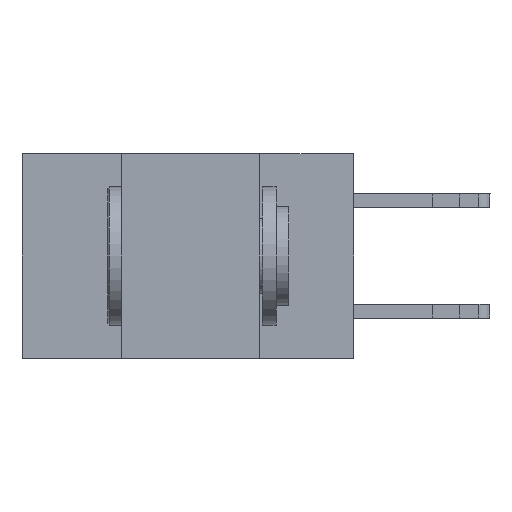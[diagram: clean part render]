
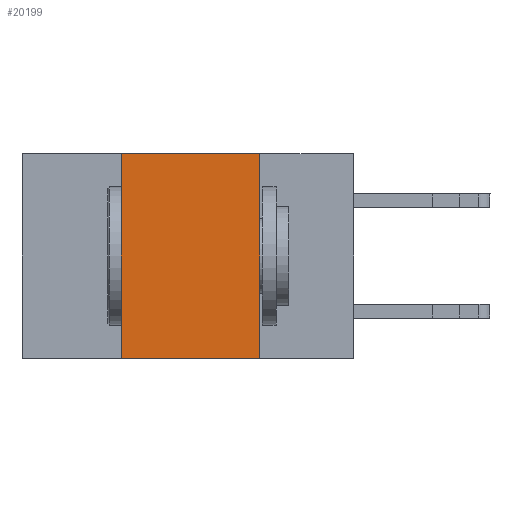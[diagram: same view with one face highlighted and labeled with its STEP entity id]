
A CAD part, left-side view. The second image highlights one B-rep face of the part: STEP entity #20199.
In plain terms, the highlighted planar face has unit normal (-1, 0, 0).
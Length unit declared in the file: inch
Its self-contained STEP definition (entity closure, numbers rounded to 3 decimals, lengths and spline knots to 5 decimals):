
#321 = PLANE ( 'NONE',  #13022 ) ;
#457 = CARTESIAN_POINT ( 'NONE',  ( 0., 0.17, -0.37 ) ) ;
#1459 = DIRECTION ( 'NONE',  ( 0., -1., 0. ) ) ;
#2272 = VERTEX_POINT ( 'NONE', #10767 ) ;
#2570 = DIRECTION ( 'NONE',  ( 1., 0., 0. ) ) ;
#2730 = CARTESIAN_POINT ( 'NONE',  ( 0., 0.17, 0. ) ) ;
#2956 = LINE ( 'NONE', #11340, #7273 ) ;
#3131 = LINE ( 'NONE', #12215, #18068 ) ;
#4416 = VECTOR ( 'NONE', #21089, 39.37008 ) ;
#4580 = EDGE_CURVE ( 'NONE', #12915, #20839, #3131, .T. ) ;
#4946 = CARTESIAN_POINT ( 'NONE',  ( 0., 0.42, 0. ) ) ;
#5567 = LINE ( 'NONE', #2730, #7060 ) ;
#6521 = CARTESIAN_POINT ( 'NONE',  ( 0., 0.6, 0. ) ) ;
#7060 = VECTOR ( 'NONE', #10227, 39.37008 ) ;
#7273 = VECTOR ( 'NONE', #1459, 39.37008 ) ;
#9674 = LINE ( 'NONE', #13425, #4416 ) ;
#9682 = CARTESIAN_POINT ( 'NONE',  ( 0., 0.42, -0.37 ) ) ;
#10227 = DIRECTION ( 'NONE',  ( 0., 0., -1. ) ) ;
#10244 = ORIENTED_EDGE ( 'NONE', *, *, #13950, .F. ) ;
#10767 = CARTESIAN_POINT ( 'NONE',  ( 0., 0.17, 0. ) ) ;
#11340 = CARTESIAN_POINT ( 'NONE',  ( 0., 0.6, 0. ) ) ;
#12215 = CARTESIAN_POINT ( 'NONE',  ( 0., 0.6, -0.37 ) ) ;
#12915 = VERTEX_POINT ( 'NONE', #9682 ) ;
#13022 = AXIS2_PLACEMENT_3D ( 'NONE', #6521, #2570, #19939 ) ;
#13425 = CARTESIAN_POINT ( 'NONE',  ( 0., 0.42, 0. ) ) ;
#13950 = EDGE_CURVE ( 'NONE', #19015, #2272, #2956, .T. ) ;
#14674 = EDGE_CURVE ( 'NONE', #12915, #19015, #9674, .T. ) ;
#14960 = ORIENTED_EDGE ( 'NONE', *, *, #18806, .F. ) ;
#18068 = VECTOR ( 'NONE', #21812, 39.37008 ) ;
#18806 = EDGE_CURVE ( 'NONE', #2272, #20839, #5567, .T. ) ;
#19015 = VERTEX_POINT ( 'NONE', #4946 ) ;
#19890 = EDGE_LOOP ( 'NONE', ( #14960, #10244, #24963, #21073 ) ) ;
#19939 = DIRECTION ( 'NONE',  ( 0., 0., -1. ) ) ;
#20199 = ADVANCED_FACE ( 'NONE', ( #21256 ), #321, .F. ) ;
#20839 = VERTEX_POINT ( 'NONE', #457 ) ;
#21073 = ORIENTED_EDGE ( 'NONE', *, *, #4580, .T. ) ;
#21089 = DIRECTION ( 'NONE',  ( 0., 0., 1. ) ) ;
#21256 = FACE_OUTER_BOUND ( 'NONE', #19890, .T. ) ;
#21812 = DIRECTION ( 'NONE',  ( 0., -1., 0. ) ) ;
#24963 = ORIENTED_EDGE ( 'NONE', *, *, #14674, .F. ) ;
